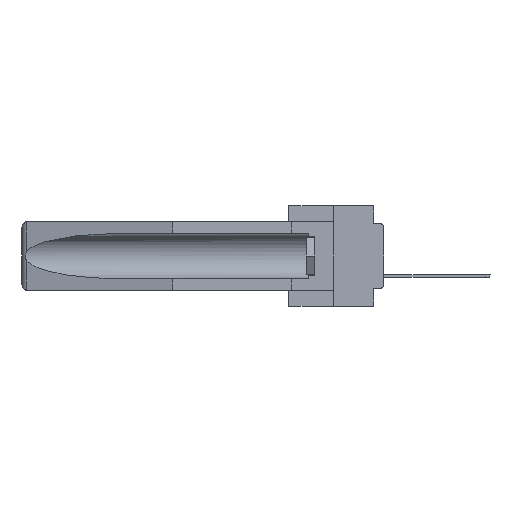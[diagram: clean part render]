
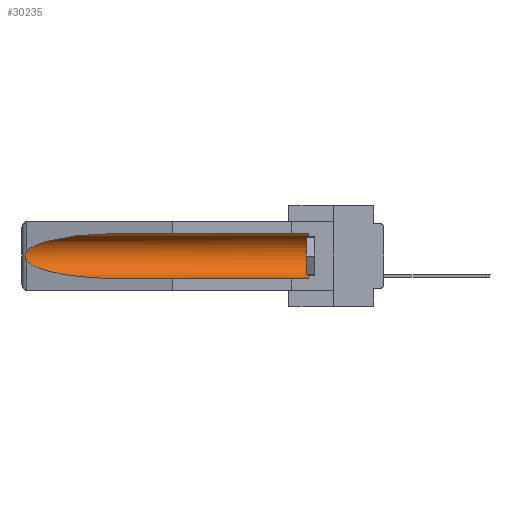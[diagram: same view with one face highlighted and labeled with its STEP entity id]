
A CAD part, left-side view. The second image highlights one B-rep face of the part: STEP entity #30235.
In plain terms, the highlighted cylindrical face has radius 2.857 mm (diameter 5.715 mm), a partial arc.
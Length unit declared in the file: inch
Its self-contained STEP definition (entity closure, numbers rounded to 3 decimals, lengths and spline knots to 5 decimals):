
#83 = DIRECTION ( 'NONE',  ( 0., 0., 1. ) ) ;
#470 = CARTESIAN_POINT ( 'NONE',  ( 0.26537, 1.52718, -0.14972 ) ) ;
#2781 = LINE ( 'NONE', #14156, #18677 ) ;
#5426 = VECTOR ( 'NONE', #10055, 39.37008 ) ;
#6184 = CARTESIAN_POINT ( 'NONE',  ( 0.2673, 1.5327, -0.16383 ) ) ;
#7773 = ORIENTED_EDGE ( 'NONE', *, *, #21135, .T. ) ;
#8357 = VERTEX_POINT ( 'NONE', #31773 ) ;
#8450 = VERTEX_POINT ( 'NONE', #26987 ) ;
#8608 = B_SPLINE_CURVE_WITH_KNOTS ( 'NONE', 3,
 ( #470, #18105, #35204, #6184, #29208, #26624, #29333, #20668, #32502, #20426 ),
 .UNSPECIFIED., .F., .F.,
 ( 4, 2, 2, 2, 4 ),
 ( 0., 0.00029, 0.00058, 0.00087, 0.00117 ),
 .UNSPECIFIED. ) ;
#8802 = CARTESIAN_POINT ( 'NONE',  ( 0.155, 0.126, -0.1715 ) ) ;
#9665 = AXIS2_PLACEMENT_3D ( 'NONE', #31044, #25381, #33590 ) ;
#9747 = CARTESIAN_POINT ( 'NONE',  ( 0.21114, 1.30732, -0.059 ) ) ;
#10055 = DIRECTION ( 'NONE',  ( 0., 1., 0. ) ) ;
#10640 = AXIS2_PLACEMENT_3D ( 'NONE', #8802, #29318, #83 ) ;
#10650 = CYLINDRICAL_SURFACE ( 'NONE', #9665, 0.1125 ) ;
#10677 = VERTEX_POINT ( 'NONE', #24317 ) ;
#12547 = CARTESIAN_POINT ( 'NONE',  ( 0.26537, 1.52718, -0.14972 ) ) ;
#14048 = LINE ( 'NONE', #33145, #5426 ) ;
#14156 = CARTESIAN_POINT ( 'NONE',  ( 0.155, -0.30754, -0.284 ) ) ;
#15888 = ORIENTED_EDGE ( 'NONE', *, *, #17590, .T. ) ;
#15938 = VERTEX_POINT ( 'NONE', #26957 ) ;
#17590 = EDGE_CURVE ( 'NONE', #31249, #10677, #35708, .T. ) ;
#18083 = EDGE_LOOP ( 'NONE', ( #15888, #25512, #7773, #24015, #18197, #24995 ) ) ;
#18105 = CARTESIAN_POINT ( 'NONE',  ( 0.26597, 1.52961, -0.15275 ) ) ;
#18156 = CARTESIAN_POINT ( 'NONE',  ( 0.155, 1.07973, -0.059 ) ) ;
#18197 = ORIENTED_EDGE ( 'NONE', *, *, #35364, .T. ) ;
#18677 = VECTOR ( 'NONE', #34600, 39.37008 ) ;
#20426 = CARTESIAN_POINT ( 'NONE',  ( 0.26537, 1.52718, -0.19328 ) ) ;
#20668 = CARTESIAN_POINT ( 'NONE',  ( 0.26655, 1.53094, -0.18657 ) ) ;
#21135 = EDGE_CURVE ( 'NONE', #8450, #8357, #36911, .T. ) ;
#21443 = CARTESIAN_POINT ( 'NONE',  ( 0.155, 0.126, -0.284 ) ) ;
#21617 = CARTESIAN_POINT ( 'NONE',  ( 0.155, 1.07973, -0.284 ) ) ;
#21802 = EDGE_CURVE ( 'NONE', #15938, #31249, #14048, .T. ) ;
#24015 = ORIENTED_EDGE ( 'NONE', *, *, #32078, .F. ) ;
#24317 = CARTESIAN_POINT ( 'NONE',  ( 0.26537, 1.52718, -0.14972 ) ) ;
#24995 = ORIENTED_EDGE ( 'NONE', *, *, #21802, .T. ) ;
#25381 = DIRECTION ( 'NONE',  ( 0., 1., 0. ) ) ;
#25512 = ORIENTED_EDGE ( 'NONE', *, *, #26443, .T. ) ;
#26443 = EDGE_CURVE ( 'NONE', #10677, #8450, #8608, .T. ) ;
#26624 = CARTESIAN_POINT ( 'NONE',  ( 0.2675, 1.53308, -0.17534 ) ) ;
#26957 = CARTESIAN_POINT ( 'NONE',  ( 0.155, 0.126, -0.059 ) ) ;
#26962 = CARTESIAN_POINT ( 'NONE',  ( 0.155, 1.07973, -0.059 ) ) ;
#26987 = CARTESIAN_POINT ( 'NONE',  ( 0.26537, 1.52718, -0.19328 ) ) ;
#27462 = CARTESIAN_POINT ( 'NONE',  ( 0.25451, 1.48313, -0.24835 ) ) ;
#29208 = CARTESIAN_POINT ( 'NONE',  ( 0.2675, 1.53308, -0.16763 ) ) ;
#29318 = DIRECTION ( 'NONE',  ( 0., -1., 0. ) ) ;
#29333 = CARTESIAN_POINT ( 'NONE',  ( 0.2673, 1.53269, -0.17917 ) ) ;
#30052 = VERTEX_POINT ( 'NONE', #21443 ) ;
#30235 = ADVANCED_FACE ( 'NONE', ( #34362 ), #10650, .F. ) ;
#30420 = CARTESIAN_POINT ( 'NONE',  ( 0.26537, 1.52718, -0.19328 ) ) ;
#30645 = CIRCLE ( 'NONE', #10640, 0.1125 ) ;
#31044 = CARTESIAN_POINT ( 'NONE',  ( 0.155, -0.30754, -0.1715 ) ) ;
#31249 = VERTEX_POINT ( 'NONE', #18156 ) ;
#31773 = CARTESIAN_POINT ( 'NONE',  ( 0.155, 1.07973, -0.284 ) ) ;
#32078 = EDGE_CURVE ( 'NONE', #30052, #8357, #2781, .T. ) ;
#32502 = CARTESIAN_POINT ( 'NONE',  ( 0.26597, 1.5296, -0.19026 ) ) ;
#32698 = CARTESIAN_POINT ( 'NONE',  ( 0.25451, 1.48313, -0.09465 ) ) ;
#33145 = CARTESIAN_POINT ( 'NONE',  ( 0.155, -0.30754, -0.059 ) ) ;
#33216 = CARTESIAN_POINT ( 'NONE',  ( 0.21114, 1.30732, -0.284 ) ) ;
#33590 = DIRECTION ( 'NONE',  ( 0., 0., 1. ) ) ;
#34362 = FACE_OUTER_BOUND ( 'NONE', #18083, .T. ) ;
#34600 = DIRECTION ( 'NONE',  ( 0., 1., 0. ) ) ;
#35204 = CARTESIAN_POINT ( 'NONE',  ( 0.26654, 1.53092, -0.15636 ) ) ;
#35364 = EDGE_CURVE ( 'NONE', #30052, #15938, #30645, .T. ) ;
#35708 =( BOUNDED_CURVE ( )  B_SPLINE_CURVE ( 3, ( #26962, #9747, #32698, #12547 ),
 .UNSPECIFIED., .F., .F. ) 
 B_SPLINE_CURVE_WITH_KNOTS ( ( 4, 4 ),
 ( 4.71239, 6.08839 ),
 .UNSPECIFIED. ) 
 CURVE ( )  GEOMETRIC_REPRESENTATION_ITEM ( )  RATIONAL_B_SPLINE_CURVE ( ( 1., 0.848, 0.848, 1. ) ) 
 REPRESENTATION_ITEM ( '' )  );
#36911 =( BOUNDED_CURVE ( )  B_SPLINE_CURVE ( 3, ( #30420, #27462, #33216, #21617 ),
 .UNSPECIFIED., .F., .F. ) 
 B_SPLINE_CURVE_WITH_KNOTS ( ( 4, 4 ),
 ( 0.1948, 1.5708 ),
 .UNSPECIFIED. ) 
 CURVE ( )  GEOMETRIC_REPRESENTATION_ITEM ( )  RATIONAL_B_SPLINE_CURVE ( ( 1., 0.848, 0.848, 1. ) ) 
 REPRESENTATION_ITEM ( '' )  );
